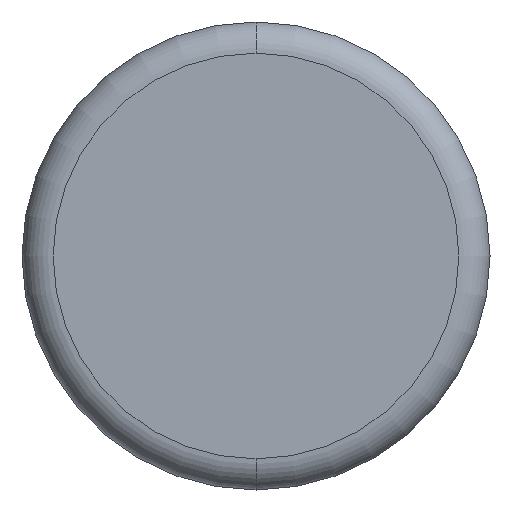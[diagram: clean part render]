
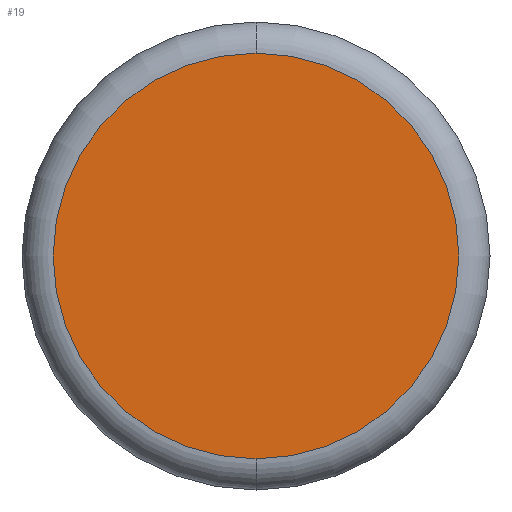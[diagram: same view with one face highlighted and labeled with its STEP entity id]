
A CAD part, front view. The second image highlights one B-rep face of the part: STEP entity #19.
In plain terms, the highlighted planar face has unit normal (0, -1, 0).
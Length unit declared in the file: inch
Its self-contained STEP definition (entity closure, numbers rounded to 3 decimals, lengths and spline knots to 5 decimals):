
#7 = ORIENTED_EDGE ( 'NONE', *, *, #101, .T. ) ;
#16 = ORIENTED_EDGE ( 'NONE', *, *, #46, .T. ) ;
#19 = ADVANCED_FACE ( 'NONE', ( #218 ), #67, .F. ) ;
#27 = VERTEX_POINT ( 'NONE', #150 ) ;
#46 = EDGE_CURVE ( 'NONE', #27, #228, #73, .T. ) ;
#48 = CARTESIAN_POINT ( 'NONE',  ( 0., 0., 0. ) ) ;
#53 = DIRECTION ( 'NONE',  ( 0., -1., 0. ) ) ;
#64 = DIRECTION ( 'NONE',  ( 0., 1., 0. ) ) ;
#67 = PLANE ( 'NONE',  #83 ) ;
#71 = CARTESIAN_POINT ( 'NONE',  ( 0., 0., 0. ) ) ;
#73 = CIRCLE ( 'NONE', #131, 0.065 ) ;
#83 = AXIS2_PLACEMENT_3D ( 'NONE', #48, #64, #106 ) ;
#101 = EDGE_CURVE ( 'NONE', #228, #27, #244, .T. ) ;
#106 = DIRECTION ( 'NONE',  ( 0., 0., 1. ) ) ;
#121 = EDGE_LOOP ( 'NONE', ( #7, #16 ) ) ;
#131 = AXIS2_PLACEMENT_3D ( 'NONE', #175, #145, #215 ) ;
#145 = DIRECTION ( 'NONE',  ( 0., -1., 0. ) ) ;
#150 = CARTESIAN_POINT ( 'NONE',  ( 0., 0., -0.065 ) ) ;
#175 = CARTESIAN_POINT ( 'NONE',  ( 0., 0., 0. ) ) ;
#188 = AXIS2_PLACEMENT_3D ( 'NONE', #71, #53, #239 ) ;
#215 = DIRECTION ( 'NONE',  ( 0., 0., 1. ) ) ;
#218 = FACE_OUTER_BOUND ( 'NONE', #121, .T. ) ;
#224 = CARTESIAN_POINT ( 'NONE',  ( 0., 0., 0.065 ) ) ;
#228 = VERTEX_POINT ( 'NONE', #224 ) ;
#239 = DIRECTION ( 'NONE',  ( 0., 0., 1. ) ) ;
#244 = CIRCLE ( 'NONE', #188, 0.065 ) ;
